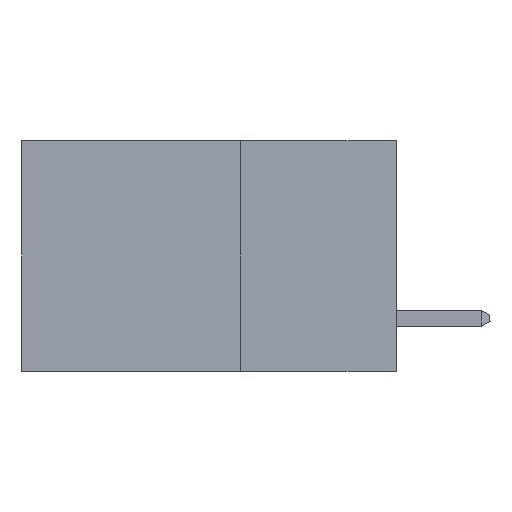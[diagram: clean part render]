
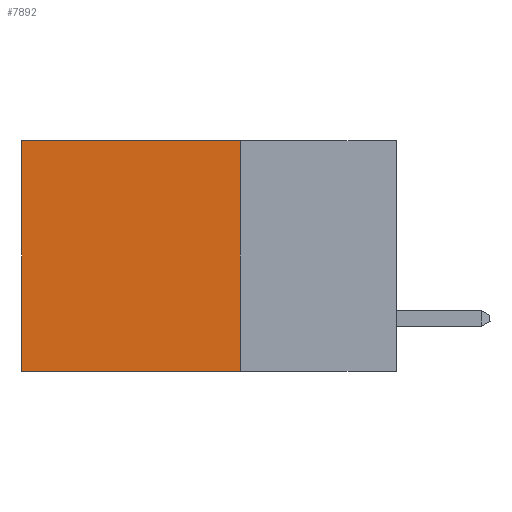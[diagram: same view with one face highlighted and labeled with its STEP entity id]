
A CAD part, left-side view. The second image highlights one B-rep face of the part: STEP entity #7892.
In plain terms, the highlighted planar face has unit normal (-1, 0, 0).
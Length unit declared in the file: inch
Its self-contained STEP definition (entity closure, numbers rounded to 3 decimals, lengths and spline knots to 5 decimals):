
#76 = DIRECTION ( 'NONE',  ( 0., 1., 0. ) ) ;
#724 = DIRECTION ( 'NONE',  ( 0., 0., -1. ) ) ;
#1100 = FACE_OUTER_BOUND ( 'NONE', #9751, .T. ) ;
#1241 = CARTESIAN_POINT ( 'NONE',  ( 0.298, 0.6, 0. ) ) ;
#1393 = ORIENTED_EDGE ( 'NONE', *, *, #8265, .T. ) ;
#1542 = AXIS2_PLACEMENT_3D ( 'NONE', #1625, #5356, #9723 ) ;
#1625 = CARTESIAN_POINT ( 'NONE',  ( 0.298, 0.25, 0. ) ) ;
#1827 = CARTESIAN_POINT ( 'NONE',  ( 0.298, 0.25, -0.37 ) ) ;
#2279 = CARTESIAN_POINT ( 'NONE',  ( 0.298, 0.25, 0. ) ) ;
#3065 = LINE ( 'NONE', #1241, #4825 ) ;
#3089 = LINE ( 'NONE', #1827, #4852 ) ;
#3316 = CARTESIAN_POINT ( 'NONE',  ( 0.298, 0.6, -0.37 ) ) ;
#3360 = VERTEX_POINT ( 'NONE', #7731 ) ;
#4564 = VERTEX_POINT ( 'NONE', #9470 ) ;
#4825 = VECTOR ( 'NONE', #724, 39.37008 ) ;
#4852 = VECTOR ( 'NONE', #7165, 39.37008 ) ;
#4911 = PLANE ( 'NONE',  #1542 ) ;
#5020 = VERTEX_POINT ( 'NONE', #3316 ) ;
#5265 = ORIENTED_EDGE ( 'NONE', *, *, #6988, .F. ) ;
#5356 = DIRECTION ( 'NONE',  ( 1., 0., 0. ) ) ;
#5500 = VECTOR ( 'NONE', #6350, 39.37008 ) ;
#5742 = LINE ( 'NONE', #2279, #5500 ) ;
#6062 = VERTEX_POINT ( 'NONE', #8327 ) ;
#6213 = LINE ( 'NONE', #7129, #8234 ) ;
#6350 = DIRECTION ( 'NONE',  ( 0., 0., -1. ) ) ;
#6988 = EDGE_CURVE ( 'NONE', #4564, #5020, #3089, .T. ) ;
#7129 = CARTESIAN_POINT ( 'NONE',  ( 0.298, 0.25, 0. ) ) ;
#7165 = DIRECTION ( 'NONE',  ( 0., 1., 0. ) ) ;
#7731 = CARTESIAN_POINT ( 'NONE',  ( 0.298, 0.25, 0. ) ) ;
#7892 = ADVANCED_FACE ( 'NONE', ( #1100 ), #4911, .F. ) ;
#8234 = VECTOR ( 'NONE', #76, 39.37008 ) ;
#8265 = EDGE_CURVE ( 'NONE', #6062, #5020, #3065, .T. ) ;
#8327 = CARTESIAN_POINT ( 'NONE',  ( 0.298, 0.6, 0. ) ) ;
#9325 = ORIENTED_EDGE ( 'NONE', *, *, #9665, .F. ) ;
#9397 = ORIENTED_EDGE ( 'NONE', *, *, #9596, .T. ) ;
#9470 = CARTESIAN_POINT ( 'NONE',  ( 0.298, 0.25, -0.37 ) ) ;
#9596 = EDGE_CURVE ( 'NONE', #3360, #6062, #6213, .T. ) ;
#9665 = EDGE_CURVE ( 'NONE', #3360, #4564, #5742, .T. ) ;
#9723 = DIRECTION ( 'NONE',  ( 0., 0., -1. ) ) ;
#9751 = EDGE_LOOP ( 'NONE', ( #1393, #5265, #9325, #9397 ) ) ;
